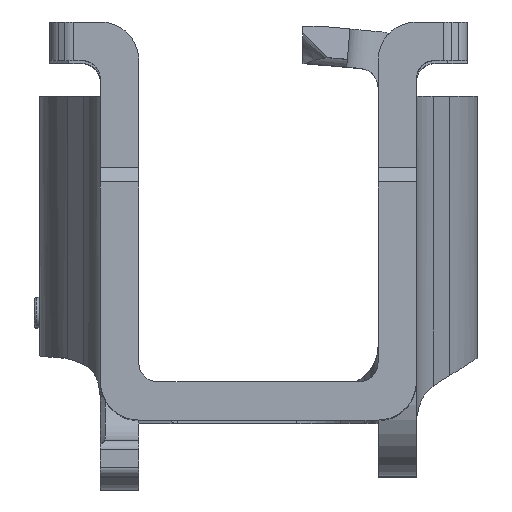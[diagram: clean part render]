
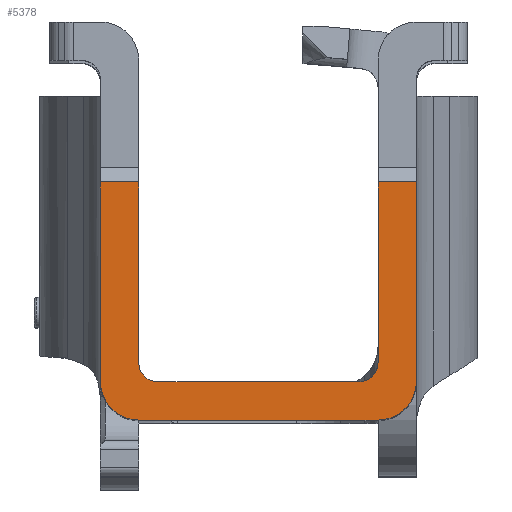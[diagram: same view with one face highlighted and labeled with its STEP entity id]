
A CAD part, top view. The second image highlights one B-rep face of the part: STEP entity #5378.
In plain terms, the highlighted planar face has unit normal (0, 0, 1).
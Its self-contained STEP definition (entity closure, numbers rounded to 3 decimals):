
#236=PLANE('',#5925);
#505=FACE_OUTER_BOUND('',#807,.T.);
#807=EDGE_LOOP('',(#4972,#4973,#4974,#4975,#4976,#4977,#4978,#4979,#4980,
#4981,#4982,#4983));
#902=CIRCLE('',#5544,1.);
#903=CIRCLE('',#5546,1.);
#1023=CIRCLE('',#5874,2.);
#1024=CIRCLE('',#5882,2.);
#1112=LINE('',#7810,#1614);
#1402=LINE('',#8963,#1904);
#1409=LINE('',#8988,#1911);
#1417=LINE('',#9005,#1919);
#1418=LINE('',#9008,#1920);
#1428=LINE('',#9076,#1930);
#1454=LINE('',#9157,#1956);
#1494=LINE('',#9278,#1996);
#1614=VECTOR('',#6172,10.);
#1904=VECTOR('',#7050,10.);
#1911=VECTOR('',#7075,10.);
#1919=VECTOR('',#7089,10.);
#1920=VECTOR('',#7092,10.);
#1930=VECTOR('',#7140,10.);
#1956=VECTOR('',#7242,10.);
#1996=VECTOR('',#7378,10.);
#2178=VERTEX_POINT('',#7807);
#2179=VERTEX_POINT('',#7809);
#2264=VERTEX_POINT('',#8082);
#2265=VERTEX_POINT('',#8086);
#2266=VERTEX_POINT('',#8088);
#2525=VERTEX_POINT('',#8961);
#2533=VERTEX_POINT('',#8985);
#2534=VERTEX_POINT('',#8987);
#2541=VERTEX_POINT('',#9007);
#2554=VERTEX_POINT('',#9075);
#2587=VERTEX_POINT('',#9250);
#2588=VERTEX_POINT('',#9274);
#2729=EDGE_CURVE('',#2179,#2178,#1112,.T.);
#2840=EDGE_CURVE('',#2264,#2178,#902,.T.);
#2842=EDGE_CURVE('',#2265,#2266,#903,.T.);
#3213=EDGE_CURVE('',#2265,#2525,#1402,.T.);
#3224=EDGE_CURVE('',#2534,#2533,#1409,.T.);
#3234=EDGE_CURVE('',#2525,#2534,#1417,.T.);
#3235=EDGE_CURVE('',#2541,#2179,#1418,.T.);
#3259=EDGE_CURVE('',#2554,#2541,#1428,.T.);
#3297=EDGE_CURVE('',#2264,#2266,#1454,.T.);
#3345=EDGE_CURVE('',#2587,#2533,#1023,.T.);
#3350=EDGE_CURVE('',#2554,#2588,#1024,.T.);
#3352=EDGE_CURVE('',#2587,#2588,#1494,.T.);
#4972=ORIENTED_EDGE('',*,*,#3235,.T.);
#4973=ORIENTED_EDGE('',*,*,#2729,.T.);
#4974=ORIENTED_EDGE('',*,*,#2840,.F.);
#4975=ORIENTED_EDGE('',*,*,#3297,.T.);
#4976=ORIENTED_EDGE('',*,*,#2842,.F.);
#4977=ORIENTED_EDGE('',*,*,#3213,.T.);
#4978=ORIENTED_EDGE('',*,*,#3234,.T.);
#4979=ORIENTED_EDGE('',*,*,#3224,.T.);
#4980=ORIENTED_EDGE('',*,*,#3345,.F.);
#4981=ORIENTED_EDGE('',*,*,#3352,.T.);
#4982=ORIENTED_EDGE('',*,*,#3350,.F.);
#4983=ORIENTED_EDGE('',*,*,#3259,.T.);
#5378=ADVANCED_FACE('',(#505),#236,.T.);
#5544=AXIS2_PLACEMENT_3D('',#8084,#6374,#6375);
#5546=AXIS2_PLACEMENT_3D('',#8089,#6379,#6380);
#5874=AXIS2_PLACEMENT_3D('',#9252,#7355,#7356);
#5882=AXIS2_PLACEMENT_3D('',#9275,#7373,#7374);
#5925=AXIS2_PLACEMENT_3D('',#9354,#7494,#7495);
#6172=DIRECTION('',(0.,-1.,0.));
#6374=DIRECTION('center_axis',(0.,0.,1.));
#6375=DIRECTION('ref_axis',(0.707,-0.707,0.));
#6379=DIRECTION('center_axis',(0.,0.,1.));
#6380=DIRECTION('ref_axis',(-0.707,-0.707,0.));
#7050=DIRECTION('',(0.,1.,0.));
#7075=DIRECTION('',(0.,-1.,0.));
#7089=DIRECTION('',(-1.,0.,0.));
#7092=DIRECTION('',(-1.,0.,0.));
#7140=DIRECTION('',(0.,1.,0.));
#7242=DIRECTION('',(-1.,0.,0.));
#7355=DIRECTION('center_axis',(0.,0.,-1.));
#7356=DIRECTION('ref_axis',(-0.707,-0.707,0.));
#7373=DIRECTION('center_axis',(0.,0.,-1.));
#7374=DIRECTION('ref_axis',(0.707,-0.707,0.));
#7378=DIRECTION('',(1.,0.,0.));
#7494=DIRECTION('center_axis',(0.,0.,1.));
#7495=DIRECTION('ref_axis',(1.,0.,0.));
#7807=CARTESIAN_POINT('',(6.25,-15.8,110.25));
#7809=CARTESIAN_POINT('',(6.25,-6.36,110.25));
#7810=CARTESIAN_POINT('',(6.25,-1.81,110.25));
#8082=CARTESIAN_POINT('',(5.25,-16.8,110.25));
#8084=CARTESIAN_POINT('Origin',(5.25,-15.8,110.25));
#8086=CARTESIAN_POINT('',(-6.25,-15.8,110.25));
#8088=CARTESIAN_POINT('',(-5.25,-16.8,110.25));
#8089=CARTESIAN_POINT('Origin',(-5.25,-15.8,110.25));
#8961=CARTESIAN_POINT('',(-6.25,-6.36,110.25));
#8963=CARTESIAN_POINT('',(-6.25,-16.8,110.25));
#8985=CARTESIAN_POINT('',(-8.25,-16.8,110.25));
#8987=CARTESIAN_POINT('',(-8.25,-6.36,110.25));
#8988=CARTESIAN_POINT('',(-8.25,-1.81,110.25));
#9005=CARTESIAN_POINT('',(4.125,-6.36,110.25));
#9007=CARTESIAN_POINT('',(8.25,-6.36,110.25));
#9008=CARTESIAN_POINT('',(4.125,-6.36,110.25));
#9075=CARTESIAN_POINT('',(8.25,-16.8,110.25));
#9076=CARTESIAN_POINT('',(8.25,-18.8,110.25));
#9157=CARTESIAN_POINT('',(6.25,-16.8,110.25));
#9250=CARTESIAN_POINT('',(-6.25,-18.8,110.25));
#9252=CARTESIAN_POINT('Origin',(-6.25,-16.8,110.25));
#9274=CARTESIAN_POINT('',(6.25,-18.8,110.25));
#9275=CARTESIAN_POINT('Origin',(6.25,-16.8,110.25));
#9278=CARTESIAN_POINT('',(-8.25,-18.8,110.25));
#9354=CARTESIAN_POINT('Origin',(0.,-10.305,110.25));
